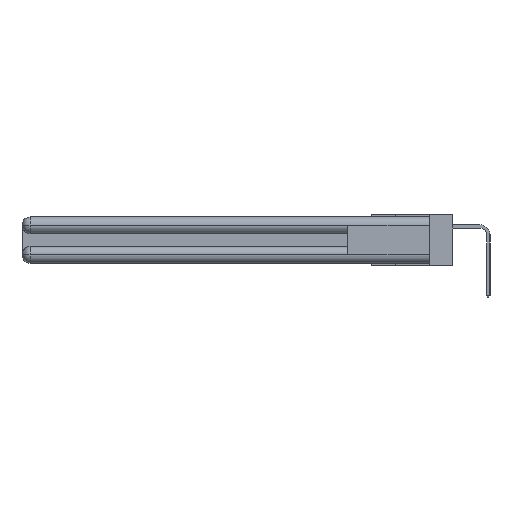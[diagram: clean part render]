
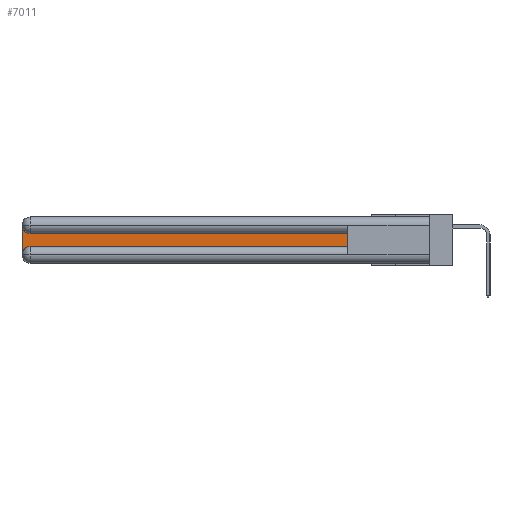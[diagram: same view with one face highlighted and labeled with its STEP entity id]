
A CAD part, left-side view. The second image highlights one B-rep face of the part: STEP entity #7011.
In plain terms, the highlighted planar face has unit normal (-1, 0, 0).
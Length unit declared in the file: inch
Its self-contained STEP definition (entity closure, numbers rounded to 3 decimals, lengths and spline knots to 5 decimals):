
#706 = DIRECTION ( 'NONE',  ( 0., 0., -1. ) ) ;
#810 = CARTESIAN_POINT ( 'NONE',  ( 0.075, 3., -0.2175 ) ) ;
#1106 = ORIENTED_EDGE ( 'NONE', *, *, #5670, .T. ) ;
#1467 = CIRCLE ( 'NONE', #21713, 0.06 ) ;
#2882 = DIRECTION ( 'NONE',  ( 0., 0., -1. ) ) ;
#3030 = VERTEX_POINT ( 'NONE', #20652 ) ;
#3057 = DIRECTION ( 'NONE',  ( 1., 0., 0. ) ) ;
#3259 = CIRCLE ( 'NONE', #14299, 0.06 ) ;
#3408 = EDGE_CURVE ( 'NONE', #7581, #21603, #27420, .T. ) ;
#4762 = EDGE_CURVE ( 'NONE', #23783, #22026, #18260, .T. ) ;
#4893 = VECTOR ( 'NONE', #706, 39.37008 ) ;
#5289 = DIRECTION ( 'NONE',  ( 0., 0., -1. ) ) ;
#5670 = EDGE_CURVE ( 'NONE', #3030, #7581, #10146, .T. ) ;
#5885 = CARTESIAN_POINT ( 'NONE',  ( 0.075, 3., -0.0625 ) ) ;
#6457 = VECTOR ( 'NONE', #9581, 39.37008 ) ;
#7011 = ADVANCED_FACE ( 'NONE', ( #29550 ), #10170, .F. ) ;
#7581 = VERTEX_POINT ( 'NONE', #20212 ) ;
#8057 = LINE ( 'NONE', #24284, #6457 ) ;
#8585 = ORIENTED_EDGE ( 'NONE', *, *, #4762, .T. ) ;
#9581 = DIRECTION ( 'NONE',  ( 0., -1., 0. ) ) ;
#9759 = CARTESIAN_POINT ( 'NONE',  ( 0.075, 0.6, -0.1225 ) ) ;
#10054 = CARTESIAN_POINT ( 'NONE',  ( 0.075, 0.6, -0.2175 ) ) ;
#10146 = LINE ( 'NONE', #10054, #16783 ) ;
#10170 = PLANE ( 'NONE',  #31790 ) ;
#10898 = ORIENTED_EDGE ( 'NONE', *, *, #31221, .T. ) ;
#11490 = CARTESIAN_POINT ( 'NONE',  ( 0.075, 2.94, -0.2175 ) ) ;
#13351 = ORIENTED_EDGE ( 'NONE', *, *, #16230, .T. ) ;
#14299 = AXIS2_PLACEMENT_3D ( 'NONE', #20240, #22732, #5289 ) ;
#14613 = DIRECTION ( 'NONE',  ( 0., 1., 0. ) ) ;
#16230 = EDGE_CURVE ( 'NONE', #22026, #23350, #3259, .T. ) ;
#16783 = VECTOR ( 'NONE', #22189, 39.37008 ) ;
#17860 = DIRECTION ( 'NONE',  ( 1., 0., 0. ) ) ;
#18248 = DIRECTION ( 'NONE',  ( 0., 0., -1. ) ) ;
#18260 = LINE ( 'NONE', #810, #4893 ) ;
#18424 = EDGE_LOOP ( 'NONE', ( #24411, #26704, #8585, #13351, #10898, #1106 ) ) ;
#20212 = CARTESIAN_POINT ( 'NONE',  ( 0.075, 0.6, -0.1225 ) ) ;
#20240 = CARTESIAN_POINT ( 'NONE',  ( 0.075, 2.94, -0.2775 ) ) ;
#20652 = CARTESIAN_POINT ( 'NONE',  ( 0.075, 0.6, -0.2175 ) ) ;
#21603 = VERTEX_POINT ( 'NONE', #24138 ) ;
#21713 = AXIS2_PLACEMENT_3D ( 'NONE', #22782, #3057, #18248 ) ;
#22026 = VERTEX_POINT ( 'NONE', #28717 ) ;
#22189 = DIRECTION ( 'NONE',  ( 0., 0., 1. ) ) ;
#22732 = DIRECTION ( 'NONE',  ( 1., 0., 0. ) ) ;
#22782 = CARTESIAN_POINT ( 'NONE',  ( 0.075, 2.94, -0.0625 ) ) ;
#23350 = VERTEX_POINT ( 'NONE', #11490 ) ;
#23783 = VERTEX_POINT ( 'NONE', #5885 ) ;
#24138 = CARTESIAN_POINT ( 'NONE',  ( 0.075, 2.94, -0.1225 ) ) ;
#24284 = CARTESIAN_POINT ( 'NONE',  ( 0.075, 0.6, -0.2175 ) ) ;
#24365 = EDGE_CURVE ( 'NONE', #21603, #23783, #1467, .T. ) ;
#24411 = ORIENTED_EDGE ( 'NONE', *, *, #3408, .T. ) ;
#26704 = ORIENTED_EDGE ( 'NONE', *, *, #24365, .T. ) ;
#27420 = LINE ( 'NONE', #9759, #27827 ) ;
#27574 = CARTESIAN_POINT ( 'NONE',  ( 0.075, 3., -0.1225 ) ) ;
#27827 = VECTOR ( 'NONE', #14613, 39.37008 ) ;
#28717 = CARTESIAN_POINT ( 'NONE',  ( 0.075, 3., -0.2775 ) ) ;
#29550 = FACE_OUTER_BOUND ( 'NONE', #18424, .T. ) ;
#31221 = EDGE_CURVE ( 'NONE', #23350, #3030, #8057, .T. ) ;
#31790 = AXIS2_PLACEMENT_3D ( 'NONE', #27574, #17860, #2882 ) ;
